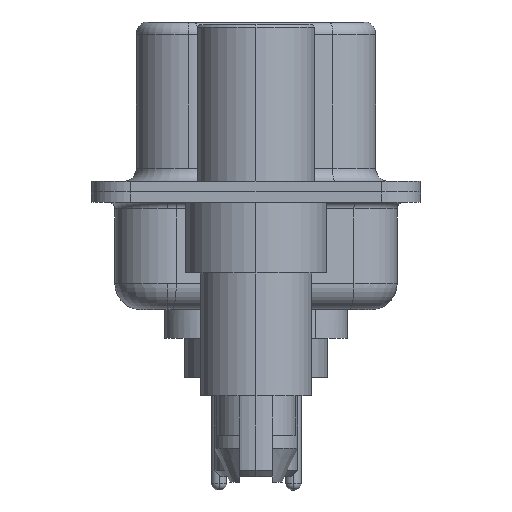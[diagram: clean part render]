
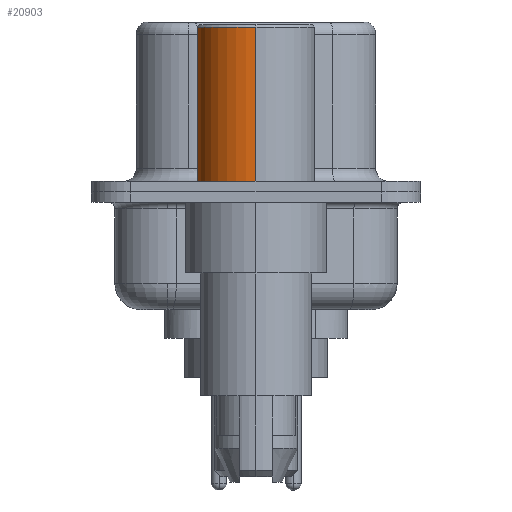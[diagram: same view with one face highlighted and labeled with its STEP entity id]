
A CAD part, left-side view. The second image highlights one B-rep face of the part: STEP entity #20903.
In plain terms, the highlighted cylindrical face has radius 2.25 mm (diameter 4.5 mm), a partial arc.
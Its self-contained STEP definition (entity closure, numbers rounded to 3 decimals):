
#668 = ORIENTED_EDGE ( 'NONE', *, *, #3898, .F. ) ;
#775 = CARTESIAN_POINT ( 'NONE',  ( -2.25, 0., 6.3 ) ) ;
#1397 = ORIENTED_EDGE ( 'NONE', *, *, #11216, .T. ) ;
#1443 = VECTOR ( 'NONE', #12183, 1000. ) ;
#1593 = CARTESIAN_POINT ( 'NONE',  ( -2.25, 0., 0.4 ) ) ;
#1956 = DIRECTION ( 'NONE',  ( 0., 0., 1. ) ) ;
#2853 = LINE ( 'NONE', #3747, #7498 ) ;
#3483 = CYLINDRICAL_SURFACE ( 'NONE', #5443, 2.25 ) ;
#3747 = CARTESIAN_POINT ( 'NONE',  ( 2.25, 0., 0.581 ) ) ;
#3898 = EDGE_CURVE ( 'NONE', #5771, #4513, #20637, .T. ) ;
#3934 = DIRECTION ( 'NONE',  ( 1., 0., 0. ) ) ;
#4073 = EDGE_LOOP ( 'NONE', ( #16251, #1397, #668, #10353 ) ) ;
#4513 = VERTEX_POINT ( 'NONE', #775 ) ;
#5375 = FACE_OUTER_BOUND ( 'NONE', #4073, .T. ) ;
#5443 = AXIS2_PLACEMENT_3D ( 'NONE', #21685, #14529, #3934 ) ;
#5771 = VERTEX_POINT ( 'NONE', #8946 ) ;
#6055 = CARTESIAN_POINT ( 'NONE',  ( 0., 0., 0.4 ) ) ;
#6527 = DIRECTION ( 'NONE',  ( 0., 0., 1. ) ) ;
#7201 = AXIS2_PLACEMENT_3D ( 'NONE', #6055, #20294, #9660 ) ;
#7498 = VECTOR ( 'NONE', #1956, 1000. ) ;
#8697 = VERTEX_POINT ( 'NONE', #22773 ) ;
#8946 = CARTESIAN_POINT ( 'NONE',  ( 2.25, 0., 6.3 ) ) ;
#9660 = DIRECTION ( 'NONE',  ( 1., 0., 0. ) ) ;
#10353 = ORIENTED_EDGE ( 'NONE', *, *, #17644, .F. ) ;
#10922 = EDGE_CURVE ( 'NONE', #8697, #21938, #13928, .T. ) ;
#11216 = EDGE_CURVE ( 'NONE', #21938, #4513, #22803, .T. ) ;
#12183 = DIRECTION ( 'NONE',  ( 0., 0., 1. ) ) ;
#13533 = DIRECTION ( 'NONE',  ( 1., 0., 0. ) ) ;
#13928 = CIRCLE ( 'NONE', #7201, 2.25 ) ;
#14529 = DIRECTION ( 'NONE',  ( 0., 0., 1. ) ) ;
#16251 = ORIENTED_EDGE ( 'NONE', *, *, #10922, .T. ) ;
#17644 = EDGE_CURVE ( 'NONE', #8697, #5771, #2853, .T. ) ;
#17764 = AXIS2_PLACEMENT_3D ( 'NONE', #18808, #6527, #13533 ) ;
#18808 = CARTESIAN_POINT ( 'NONE',  ( 0., 0., 6.3 ) ) ;
#20294 = DIRECTION ( 'NONE',  ( 0., 0., 1. ) ) ;
#20637 = CIRCLE ( 'NONE', #17764, 2.25 ) ;
#20903 = ADVANCED_FACE ( 'NONE', ( #5375 ), #3483, .T. ) ;
#20971 = CARTESIAN_POINT ( 'NONE',  ( -2.25, 0., 0.581 ) ) ;
#21685 = CARTESIAN_POINT ( 'NONE',  ( 0., 0., 0.581 ) ) ;
#21938 = VERTEX_POINT ( 'NONE', #1593 ) ;
#22773 = CARTESIAN_POINT ( 'NONE',  ( 2.25, 0., 0.4 ) ) ;
#22803 = LINE ( 'NONE', #20971, #1443 ) ;
